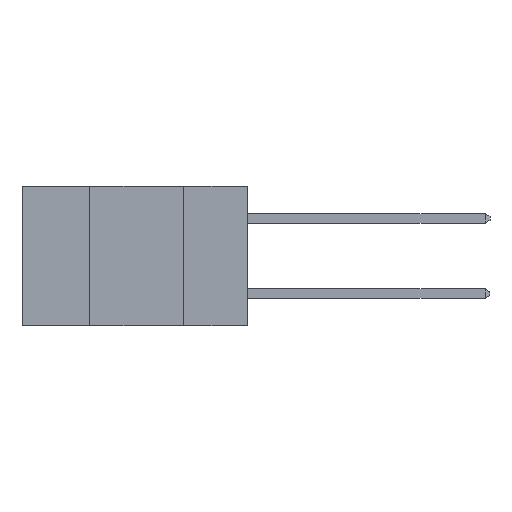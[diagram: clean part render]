
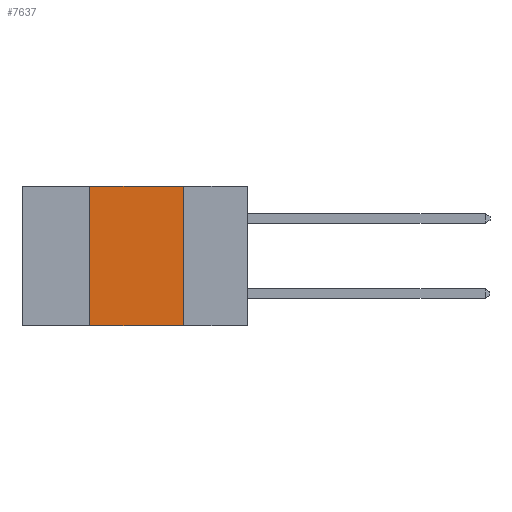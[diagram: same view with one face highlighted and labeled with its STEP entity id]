
A CAD part, left-side view. The second image highlights one B-rep face of the part: STEP entity #7637.
In plain terms, the highlighted planar face has unit normal (-1, 0, 0).
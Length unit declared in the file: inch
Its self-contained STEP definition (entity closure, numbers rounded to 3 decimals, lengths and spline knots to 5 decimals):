
#507 = ORIENTED_EDGE ( 'NONE', *, *, #6542, .F. ) ;
#1760 = VECTOR ( 'NONE', #7878, 39.37008 ) ;
#2245 = DIRECTION ( 'NONE',  ( 0., -1., 0. ) ) ;
#3159 = VECTOR ( 'NONE', #2245, 39.37008 ) ;
#3907 = CARTESIAN_POINT ( 'NONE',  ( 0., 0.6, 0. ) ) ;
#4695 = CARTESIAN_POINT ( 'NONE',  ( 0., 0.17, 0. ) ) ;
#6154 = EDGE_CURVE ( 'NONE', #27828, #29906, #14461, .T. ) ;
#6444 = DIRECTION ( 'NONE',  ( 0., -1., 0. ) ) ;
#6542 = EDGE_CURVE ( 'NONE', #29906, #31283, #28601, .T. ) ;
#7637 = ADVANCED_FACE ( 'NONE', ( #28129 ), #14493, .F. ) ;
#7878 = DIRECTION ( 'NONE',  ( 0., 0., -1. ) ) ;
#9142 = DIRECTION ( 'NONE',  ( 0., 0., 1. ) ) ;
#9418 = CARTESIAN_POINT ( 'NONE',  ( 0., 0.6, 0. ) ) ;
#9816 = CARTESIAN_POINT ( 'NONE',  ( 0., 0.17, -0.37 ) ) ;
#9907 = LINE ( 'NONE', #27381, #3159 ) ;
#13794 = AXIS2_PLACEMENT_3D ( 'NONE', #9418, #32063, #17033 ) ;
#14461 = LINE ( 'NONE', #3907, #27045 ) ;
#14493 = PLANE ( 'NONE',  #13794 ) ;
#16457 = CARTESIAN_POINT ( 'NONE',  ( 0., 0.42, -0.37 ) ) ;
#17033 = DIRECTION ( 'NONE',  ( 0., 0., -1. ) ) ;
#17910 = CARTESIAN_POINT ( 'NONE',  ( 0., 0.17, 0. ) ) ;
#20335 = LINE ( 'NONE', #29290, #27019 ) ;
#23039 = ORIENTED_EDGE ( 'NONE', *, *, #26816, .F. ) ;
#25396 = EDGE_LOOP ( 'NONE', ( #507, #28156, #23039, #26197 ) ) ;
#25838 = CARTESIAN_POINT ( 'NONE',  ( 0., 0.42, 0. ) ) ;
#26197 = ORIENTED_EDGE ( 'NONE', *, *, #31859, .T. ) ;
#26816 = EDGE_CURVE ( 'NONE', #30360, #27828, #20335, .T. ) ;
#27019 = VECTOR ( 'NONE', #9142, 39.37008 ) ;
#27045 = VECTOR ( 'NONE', #6444, 39.37008 ) ;
#27381 = CARTESIAN_POINT ( 'NONE',  ( 0., 0.6, -0.37 ) ) ;
#27828 = VERTEX_POINT ( 'NONE', #25838 ) ;
#28129 = FACE_OUTER_BOUND ( 'NONE', #25396, .T. ) ;
#28156 = ORIENTED_EDGE ( 'NONE', *, *, #6154, .F. ) ;
#28601 = LINE ( 'NONE', #17910, #1760 ) ;
#29290 = CARTESIAN_POINT ( 'NONE',  ( 0., 0.42, 0. ) ) ;
#29906 = VERTEX_POINT ( 'NONE', #4695 ) ;
#30360 = VERTEX_POINT ( 'NONE', #16457 ) ;
#31283 = VERTEX_POINT ( 'NONE', #9816 ) ;
#31859 = EDGE_CURVE ( 'NONE', #30360, #31283, #9907, .T. ) ;
#32063 = DIRECTION ( 'NONE',  ( 1., 0., 0. ) ) ;
